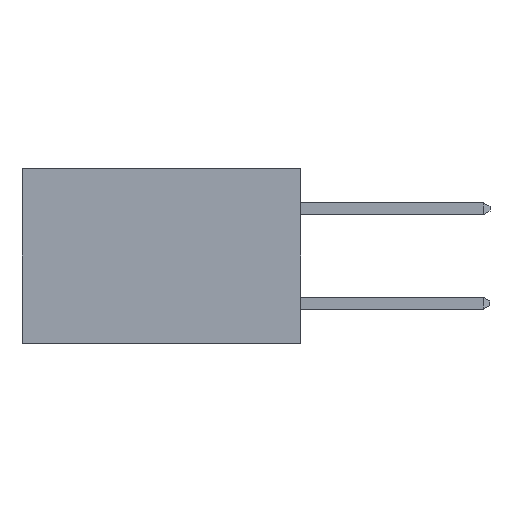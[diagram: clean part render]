
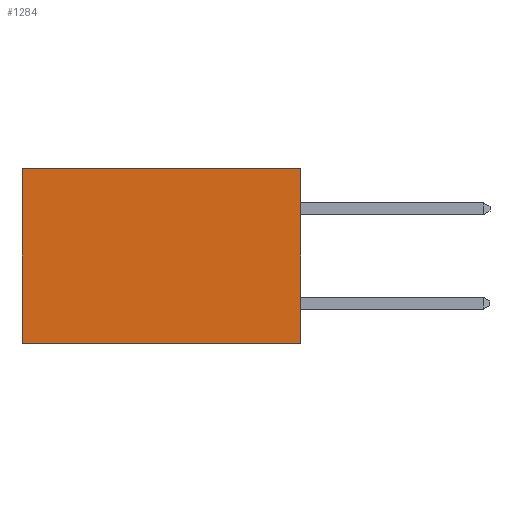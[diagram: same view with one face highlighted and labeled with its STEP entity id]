
A CAD part, left-side view. The second image highlights one B-rep face of the part: STEP entity #1284.
In plain terms, the highlighted planar face has unit normal (-1, 0, 0).
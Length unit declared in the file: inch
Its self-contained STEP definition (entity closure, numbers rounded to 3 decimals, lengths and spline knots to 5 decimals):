
#550 = VERTEX_POINT ( 'NONE', #3725 ) ;
#1234 = EDGE_CURVE ( 'NONE', #3964, #4182, #3821, .T. ) ;
#1284 = ADVANCED_FACE ( 'NONE', ( #3209 ), #8048, .F. ) ;
#1293 = EDGE_CURVE ( 'NONE', #4182, #8116, #8043, .T. ) ;
#1482 = EDGE_CURVE ( 'NONE', #3964, #550, #6468, .T. ) ;
#1633 = VECTOR ( 'NONE', #7767, 39.37008 ) ;
#1775 = ORIENTED_EDGE ( 'NONE', *, *, #1482, .F. ) ;
#2347 = DIRECTION ( 'NONE',  ( 0., 0., -1. ) ) ;
#3107 = VECTOR ( 'NONE', #2347, 39.37008 ) ;
#3209 = FACE_OUTER_BOUND ( 'NONE', #3664, .T. ) ;
#3358 = CARTESIAN_POINT ( 'NONE',  ( 0.277, 0., -0.37 ) ) ;
#3545 = ORIENTED_EDGE ( 'NONE', *, *, #1234, .T. ) ;
#3664 = EDGE_LOOP ( 'NONE', ( #5043, #8353, #1775, #3545 ) ) ;
#3725 = CARTESIAN_POINT ( 'NONE',  ( 0.277, 0., -0.37 ) ) ;
#3821 = LINE ( 'NONE', #8147, #5499 ) ;
#3964 = VERTEX_POINT ( 'NONE', #4180 ) ;
#3984 = CARTESIAN_POINT ( 'NONE',  ( 0.277, 0.59, -0.37 ) ) ;
#4180 = CARTESIAN_POINT ( 'NONE',  ( 0.277, 0., 0. ) ) ;
#4182 = VERTEX_POINT ( 'NONE', #8106 ) ;
#5043 = ORIENTED_EDGE ( 'NONE', *, *, #1293, .T. ) ;
#5284 = DIRECTION ( 'NONE',  ( 0., 1., 0. ) ) ;
#5499 = VECTOR ( 'NONE', #8113, 39.37008 ) ;
#5618 = LINE ( 'NONE', #3358, #5811 ) ;
#5803 = CARTESIAN_POINT ( 'NONE',  ( 0.277, 0., -0.37 ) ) ;
#5811 = VECTOR ( 'NONE', #5284, 39.37008 ) ;
#5871 = AXIS2_PLACEMENT_3D ( 'NONE', #7944, #7857, #7828 ) ;
#6468 = LINE ( 'NONE', #5803, #3107 ) ;
#6554 = EDGE_CURVE ( 'NONE', #550, #8116, #5618, .T. ) ;
#7762 = CARTESIAN_POINT ( 'NONE',  ( 0.277, 0.59, -0.37 ) ) ;
#7767 = DIRECTION ( 'NONE',  ( 0., 0., -1. ) ) ;
#7828 = DIRECTION ( 'NONE',  ( 0., 0., -1. ) ) ;
#7857 = DIRECTION ( 'NONE',  ( 1., 0., 0. ) ) ;
#7944 = CARTESIAN_POINT ( 'NONE',  ( 0.277, 0., -0.37 ) ) ;
#8043 = LINE ( 'NONE', #7762, #1633 ) ;
#8048 = PLANE ( 'NONE',  #5871 ) ;
#8106 = CARTESIAN_POINT ( 'NONE',  ( 0.277, 0.59, 0. ) ) ;
#8113 = DIRECTION ( 'NONE',  ( 0., 1., 0. ) ) ;
#8116 = VERTEX_POINT ( 'NONE', #3984 ) ;
#8147 = CARTESIAN_POINT ( 'NONE',  ( 0.277, 0., 0. ) ) ;
#8353 = ORIENTED_EDGE ( 'NONE', *, *, #6554, .F. ) ;
